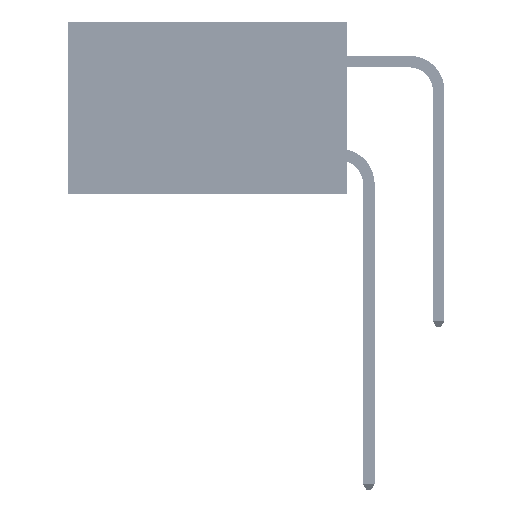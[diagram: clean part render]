
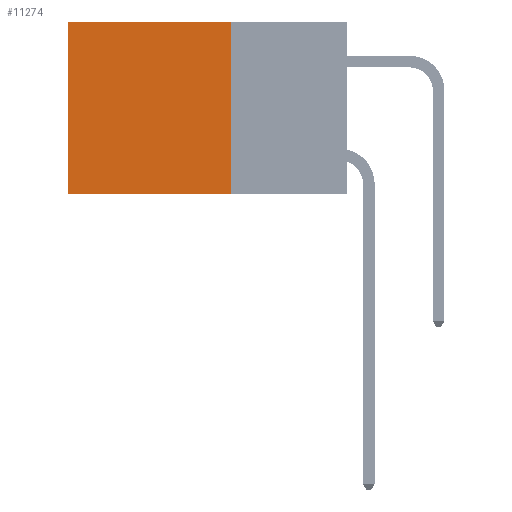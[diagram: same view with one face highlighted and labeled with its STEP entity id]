
A CAD part, left-side view. The second image highlights one B-rep face of the part: STEP entity #11274.
In plain terms, the highlighted planar face has unit normal (-1, 0, 0).
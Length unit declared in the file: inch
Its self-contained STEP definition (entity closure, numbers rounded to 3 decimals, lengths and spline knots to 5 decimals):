
#3197 = DIRECTION ( 'NONE',  ( 0., 1., 0. ) ) ;
#5694 = DIRECTION ( 'NONE',  ( 0., 0., -1. ) ) ;
#6052 = VERTEX_POINT ( 'NONE', #35564 ) ;
#7346 = EDGE_CURVE ( 'NONE', #6052, #34596, #37689, .T. ) ;
#7566 = CARTESIAN_POINT ( 'NONE',  ( 0.2875, 0.25, -0.37 ) ) ;
#7786 = VECTOR ( 'NONE', #52022, 39.37008 ) ;
#9677 = VECTOR ( 'NONE', #5694, 39.37008 ) ;
#10848 = CARTESIAN_POINT ( 'NONE',  ( 0.2875, 0.6, 0. ) ) ;
#11143 = VECTOR ( 'NONE', #28202, 39.37008 ) ;
#11274 = ADVANCED_FACE ( 'NONE', ( #40413 ), #53021, .F. ) ;
#14877 = CARTESIAN_POINT ( 'NONE',  ( 0.2875, 0.6, 0. ) ) ;
#16505 = VERTEX_POINT ( 'NONE', #26274 ) ;
#17496 = CARTESIAN_POINT ( 'NONE',  ( 0.2875, 0.25, -0.37 ) ) ;
#18604 = LINE ( 'NONE', #32291, #19942 ) ;
#19942 = VECTOR ( 'NONE', #3197, 39.37008 ) ;
#21949 = VERTEX_POINT ( 'NONE', #10848 ) ;
#26274 = CARTESIAN_POINT ( 'NONE',  ( 0.2875, 0.6, -0.37 ) ) ;
#28202 = DIRECTION ( 'NONE',  ( 0., 1., 0. ) ) ;
#30080 = ORIENTED_EDGE ( 'NONE', *, *, #7346, .F. ) ;
#30716 = LINE ( 'NONE', #7566, #11143 ) ;
#32291 = CARTESIAN_POINT ( 'NONE',  ( 0.2875, 0.25, 0. ) ) ;
#32490 = ORIENTED_EDGE ( 'NONE', *, *, #33917, .T. ) ;
#33917 = EDGE_CURVE ( 'NONE', #6052, #21949, #18604, .T. ) ;
#34596 = VERTEX_POINT ( 'NONE', #17496 ) ;
#35564 = CARTESIAN_POINT ( 'NONE',  ( 0.2875, 0.25, 0. ) ) ;
#37689 = LINE ( 'NONE', #47040, #9677 ) ;
#40413 = FACE_OUTER_BOUND ( 'NONE', #51922, .T. ) ;
#40454 = CARTESIAN_POINT ( 'NONE',  ( 0.2875, 0.25, 0. ) ) ;
#44263 = DIRECTION ( 'NONE',  ( 1., 0., 0. ) ) ;
#44527 = EDGE_CURVE ( 'NONE', #34596, #16505, #30716, .T. ) ;
#44865 = ORIENTED_EDGE ( 'NONE', *, *, #44527, .F. ) ;
#46870 = ORIENTED_EDGE ( 'NONE', *, *, #50204, .T. ) ;
#47040 = CARTESIAN_POINT ( 'NONE',  ( 0.2875, 0.25, 0. ) ) ;
#47966 = AXIS2_PLACEMENT_3D ( 'NONE', #40454, #44263, #48459 ) ;
#48459 = DIRECTION ( 'NONE',  ( 0., 0., -1. ) ) ;
#50204 = EDGE_CURVE ( 'NONE', #21949, #16505, #52126, .T. ) ;
#51922 = EDGE_LOOP ( 'NONE', ( #46870, #44865, #30080, #32490 ) ) ;
#52022 = DIRECTION ( 'NONE',  ( 0., 0., -1. ) ) ;
#52126 = LINE ( 'NONE', #14877, #7786 ) ;
#53021 = PLANE ( 'NONE',  #47966 ) ;
